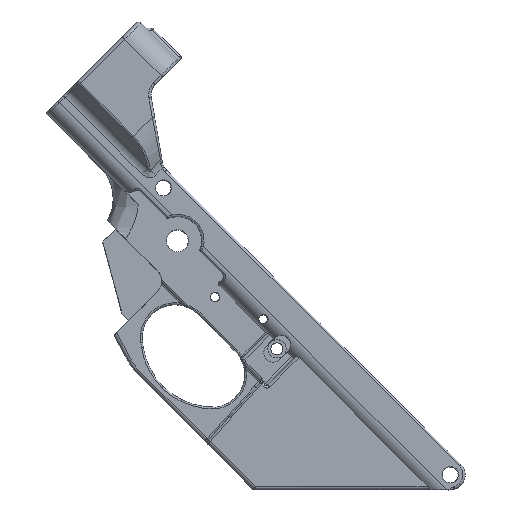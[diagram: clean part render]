
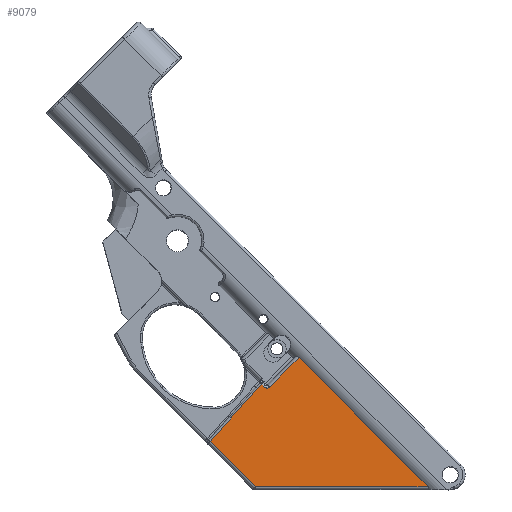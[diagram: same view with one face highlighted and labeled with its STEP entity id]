
A CAD part, front view. The second image highlights one B-rep face of the part: STEP entity #9079.
In plain terms, the highlighted planar face has unit normal (0.006, -1, 0.006).
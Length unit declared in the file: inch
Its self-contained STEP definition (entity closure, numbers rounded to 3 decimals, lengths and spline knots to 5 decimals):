
#2426 = CARTESIAN_POINT ( 'NONE',  ( 1.16658, -1.42758, -1.5382 ) ) ;
#2629 = CARTESIAN_POINT ( 'NONE',  ( 1.20017, -1.42758, -1.57179 ) ) ;
#2859 = CARTESIAN_POINT ( 'NONE',  ( 1.06101, -1.43892, -3.27011 ) ) ;
#3265 = VERTEX_POINT ( 'NONE', #16781 ) ;
#3366 = EDGE_CURVE ( 'NONE', #13884, #24815, #11044, .T. ) ;
#4077 = DIRECTION ( 'NONE',  ( -0.707, 0., 0.707 ) ) ;
#5248 = LINE ( 'NONE', #8698, #26562 ) ;
#5434 = CARTESIAN_POINT ( 'NONE',  ( 1.21554, -1.42757, -1.585 ) ) ;
#5775 = LINE ( 'NONE', #29593, #19703 ) ;
#5949 = PLANE ( 'NONE',  #25428 ) ;
#6065 = CARTESIAN_POINT ( 'NONE',  ( 1.81354, -1.4151, -0.16291 ) ) ;
#6176 = DIRECTION ( 'NONE',  ( 1., 0.006, 0. ) ) ;
#6201 = DIRECTION ( 'NONE',  ( -0.707, 0., 0.707 ) ) ;
#6269 = VECTOR ( 'NONE', #6176, 39.37008 ) ;
#7171 = EDGE_CURVE ( 'NONE', #12512, #17047, #26572, .T. ) ;
#7385 = EDGE_CURVE ( 'NONE', #24815, #35547, #5248, .T. ) ;
#7618 = EDGE_LOOP ( 'NONE', ( #19073, #29540, #24280, #16543, #13659, #25039, #15306, #19826, #23980 ) ) ;
#8025 = CARTESIAN_POINT ( 'NONE',  ( 1.09725, -1.42843, -1.60753 ) ) ;
#8224 = CARTESIAN_POINT ( 'NONE',  ( 1.23879, -1.4275, -1.59721 ) ) ;
#8307 = VECTOR ( 'NONE', #4077, 39.37008 ) ;
#8503 = CARTESIAN_POINT ( 'NONE',  ( -0.17002, -1.44494, -3.01498 ) ) ;
#8684 = VERTEX_POINT ( 'NONE', #2859 ) ;
#8698 = CARTESIAN_POINT ( 'NONE',  ( 0.13404, -1.44098, -2.67728 ) ) ;
#8869 = DIRECTION ( 'NONE',  ( -0.707, -0.009, -0.707 ) ) ;
#9079 = ADVANCED_FACE ( 'NONE', ( #22522 ), #5949, .T. ) ;
#10777 = EDGE_CURVE ( 'NONE', #23775, #3265, #29582, .T. ) ;
#11044 = LINE ( 'NONE', #8503, #19285 ) ;
#11075 = CARTESIAN_POINT ( 'NONE',  ( 1.26285, -1.42738, -1.60207 ) ) ;
#11342 = DIRECTION ( 'NONE',  ( 0.669, 0.009, 0.743 ) ) ;
#12512 = VERTEX_POINT ( 'NONE', #27662 ) ;
#13046 = VECTOR ( 'NONE', #20880, 39.37008 ) ;
#13220 = EDGE_CURVE ( 'NONE', #8684, #23775, #21059, .T. ) ;
#13659 = ORIENTED_EDGE ( 'NONE', *, *, #20437, .T. ) ;
#13814 = CARTESIAN_POINT ( 'NONE',  ( 1.28919, -1.42718, -1.5959 ) ) ;
#13884 = VERTEX_POINT ( 'NONE', #14266 ) ;
#14264 = DIRECTION ( 'NONE',  ( 0.669, 0.009, 0.743 ) ) ;
#14266 = CARTESIAN_POINT ( 'NONE',  ( 0.29236, -1.43892, -2.50145 ) ) ;
#15306 = ORIENTED_EDGE ( 'NONE', *, *, #18171, .T. ) ;
#16186 = EDGE_CURVE ( 'NONE', #13884, #8684, #34329, .T. ) ;
#16543 = ORIENTED_EDGE ( 'NONE', *, *, #10777, .T. ) ;
#16781 = CARTESIAN_POINT ( 'NONE',  ( 1.80168, -1.42085, -1.08341 ) ) ;
#17047 = VERTEX_POINT ( 'NONE', #27431 ) ;
#17235 = CARTESIAN_POINT ( 'NONE',  ( 1.8136, -1.43427, -3.27012 ) ) ;
#18171 = EDGE_CURVE ( 'NONE', #12512, #33774, #20563, .T. ) ;
#18297 = CARTESIAN_POINT ( 'NONE',  ( 2.34719, -1.42085, -1.62892 ) ) ;
#19073 = ORIENTED_EDGE ( 'NONE', *, *, #3366, .F. ) ;
#19285 = VECTOR ( 'NONE', #11342, 39.37008 ) ;
#19315 = CARTESIAN_POINT ( 'NONE',  ( 1.2078, -1.42758, -1.57942 ) ) ;
#19703 = VECTOR ( 'NONE', #24038, 39.37008 ) ;
#19826 = ORIENTED_EDGE ( 'NONE', *, *, #30628, .T. ) ;
#20437 = EDGE_CURVE ( 'NONE', #3265, #17047, #5775, .T. ) ;
#20563 = LINE ( 'NONE', #25664, #27095 ) ;
#20872 = DIRECTION ( 'NONE',  ( -0.707, -0.009, -0.707 ) ) ;
#20880 = DIRECTION ( 'NONE',  ( 0.707, 0., -0.707 ) ) ;
#20890 = CARTESIAN_POINT ( 'NONE',  ( 3.98844, -1.42085, -3.27017 ) ) ;
#21059 = LINE ( 'NONE', #17235, #6269 ) ;
#22522 = FACE_OUTER_BOUND ( 'NONE', #7618, .T. ) ;
#22619 = CARTESIAN_POINT ( 'NONE',  ( 0.64694, -1.4343, -2.10765 ) ) ;
#23775 = VERTEX_POINT ( 'NONE', #20890 ) ;
#23790 = CARTESIAN_POINT ( 'NONE',  ( -0.11632, -1.43892, -2.09278 ) ) ;
#23980 = ORIENTED_EDGE ( 'NONE', *, *, #7385, .F. ) ;
#24038 = DIRECTION ( 'NONE',  ( -0.707, -0.009, -0.707 ) ) ;
#24280 = ORIENTED_EDGE ( 'NONE', *, *, #13220, .T. ) ;
#24815 = VERTEX_POINT ( 'NONE', #22619 ) ;
#24892 = CARTESIAN_POINT ( 'NONE',  ( 1.23101, -1.42752, -1.59391 ) ) ;
#25039 = ORIENTED_EDGE ( 'NONE', *, *, #7171, .F. ) ;
#25428 = AXIS2_PLACEMENT_3D ( 'NONE', #6065, #25532, #8869 ) ;
#25532 = DIRECTION ( 'NONE',  ( 0.006, -1., 0.006 ) ) ;
#25664 = CARTESIAN_POINT ( 'NONE',  ( 0.80242, -1.42758, -1.17404 ) ) ;
#26562 = VECTOR ( 'NONE', #14264, 39.37008 ) ;
#26572 = B_SPLINE_CURVE_WITH_KNOTS ( 'NONE', 3,
 ( #2629, #19315, #5434, #24892, #8224, #27658, #11075, #30427, #13814, #33246 ),
 .UNSPECIFIED., .F., .F.,
 ( 4, 2, 2, 2, 4 ),
 ( 0., 0.25, 0.5, 0.75, 1. ),
 .UNSPECIFIED. ) ;
#26848 = VECTOR ( 'NONE', #20872, 39.37008 ) ;
#27095 = VECTOR ( 'NONE', #6201, 39.37008 ) ;
#27431 = CARTESIAN_POINT ( 'NONE',  ( 1.29916, -1.42706, -1.58593 ) ) ;
#27658 = CARTESIAN_POINT ( 'NONE',  ( 1.25471, -1.42742, -1.60127 ) ) ;
#27662 = CARTESIAN_POINT ( 'NONE',  ( 1.20017, -1.42758, -1.57179 ) ) ;
#29109 = CARTESIAN_POINT ( 'NONE',  ( 1.35352, -1.42527, -1.35126 ) ) ;
#29540 = ORIENTED_EDGE ( 'NONE', *, *, #16186, .T. ) ;
#29582 = LINE ( 'NONE', #18297, #8307 ) ;
#29593 = CARTESIAN_POINT ( 'NONE',  ( 1.29348, -1.42713, -1.59161 ) ) ;
#30427 = CARTESIAN_POINT ( 'NONE',  ( 1.28001, -1.42725, -1.59917 ) ) ;
#30628 = EDGE_CURVE ( 'NONE', #33774, #35547, #34219, .T. ) ;
#33246 = CARTESIAN_POINT ( 'NONE',  ( 1.29916, -1.42706, -1.58593 ) ) ;
#33774 = VERTEX_POINT ( 'NONE', #2426 ) ;
#34219 = LINE ( 'NONE', #29109, #26848 ) ;
#34329 = LINE ( 'NONE', #23790, #13046 ) ;
#35547 = VERTEX_POINT ( 'NONE', #8025 ) ;
